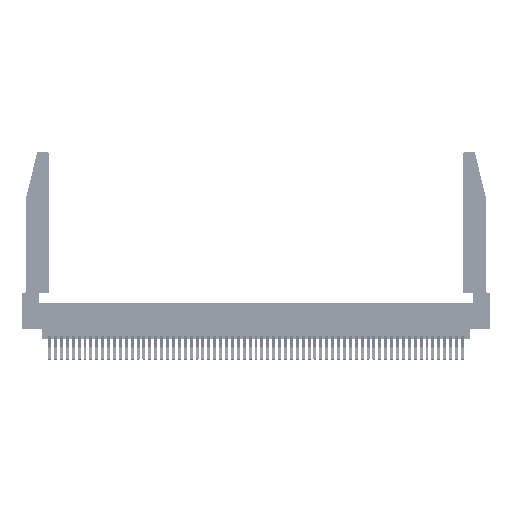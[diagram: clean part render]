
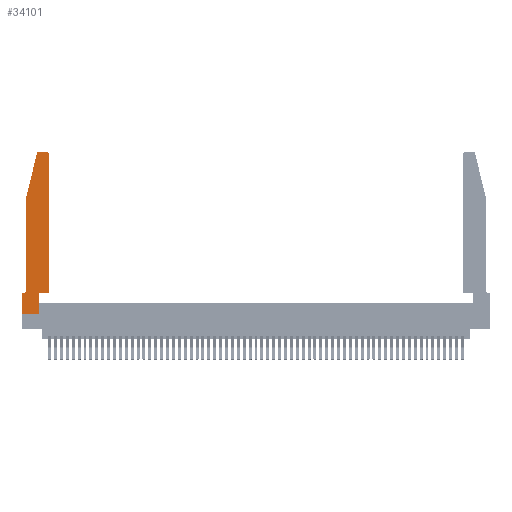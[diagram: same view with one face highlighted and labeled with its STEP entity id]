
A CAD part, top view. The second image highlights one B-rep face of the part: STEP entity #34101.
In plain terms, the highlighted planar face has unit normal (0, 0, 1).
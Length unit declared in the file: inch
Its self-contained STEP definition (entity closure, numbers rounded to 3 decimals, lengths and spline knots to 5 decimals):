
#164 = EDGE_LOOP ( 'NONE', ( #27753, #13057, #51503, #23062, #17899, #21188, #3641, #48083, #56611, #24493, #34221, #52091 ) ) ;
#1162 = LINE ( 'NONE', #53450, #11556 ) ;
#1412 = VERTEX_POINT ( 'NONE', #24696 ) ;
#2432 = CARTESIAN_POINT ( 'NONE',  ( 0.0755, 0.42, 0.37 ) ) ;
#3641 = ORIENTED_EDGE ( 'NONE', *, *, #24181, .T. ) ;
#4455 = VECTOR ( 'NONE', #11091, 39.37008 ) ;
#4553 = CARTESIAN_POINT ( 'NONE',  ( 0.4205, 2.72, 0.37 ) ) ;
#5478 = DIRECTION ( 'NONE',  ( 1., 0., 0. ) ) ;
#6006 = CARTESIAN_POINT ( 'NONE',  ( 0., 0., 0.37 ) ) ;
#6421 = EDGE_CURVE ( 'NONE', #43641, #56479, #15520, .T. ) ;
#6986 = EDGE_CURVE ( 'NONE', #33085, #43641, #43391, .T. ) ;
#7596 = DIRECTION ( 'NONE',  ( 0., 0., -1. ) ) ;
#7660 = AXIS2_PLACEMENT_3D ( 'NONE', #39767, #22393, #52934 ) ;
#7794 = VERTEX_POINT ( 'NONE', #12949 ) ;
#8035 = LINE ( 'NONE', #33126, #53197 ) ;
#8493 = VECTOR ( 'NONE', #38979, 39.37008 ) ;
#8768 = LINE ( 'NONE', #17458, #53961 ) ;
#8967 = DIRECTION ( 'NONE',  ( 1., 0., 0. ) ) ;
#10616 = LINE ( 'NONE', #17652, #33943 ) ;
#10842 = EDGE_CURVE ( 'NONE', #40890, #40761, #20466, .T. ) ;
#11091 = DIRECTION ( 'NONE',  ( 0., -1., 0. ) ) ;
#11556 = VECTOR ( 'NONE', #36266, 39.37008 ) ;
#12339 = EDGE_CURVE ( 'NONE', #35176, #49498, #49645, .T. ) ;
#12483 = EDGE_CURVE ( 'NONE', #49498, #7794, #42803, .T. ) ;
#12949 = CARTESIAN_POINT ( 'NONE',  ( 0.0055, 0.35, 0.37 ) ) ;
#13057 = ORIENTED_EDGE ( 'NONE', *, *, #10842, .T. ) ;
#15520 = CIRCLE ( 'NONE', #21879, 0.03 ) ;
#16499 = LINE ( 'NONE', #38574, #25376 ) ;
#16634 = DIRECTION ( 'NONE',  ( -1., 0., 0. ) ) ;
#16888 = DIRECTION ( 'NONE',  ( 0., 1., 0. ) ) ;
#17458 = CARTESIAN_POINT ( 'NONE',  ( 0.4505, 0.35, 0.37 ) ) ;
#17652 = CARTESIAN_POINT ( 'NONE',  ( 0., 0., 0.37 ) ) ;
#17899 = ORIENTED_EDGE ( 'NONE', *, *, #12483, .T. ) ;
#18102 = CARTESIAN_POINT ( 'NONE',  ( 0.4205, 2.75, 0.37 ) ) ;
#18366 = CARTESIAN_POINT ( 'NONE',  ( 0.284, 2.72, 0.37 ) ) ;
#18571 = CARTESIAN_POINT ( 'NONE',  ( 0., 0., 0.37 ) ) ;
#18648 = EDGE_CURVE ( 'NONE', #40761, #35176, #1162, .T. ) ;
#20393 = VECTOR ( 'NONE', #16888, 39.37008 ) ;
#20466 = CIRCLE ( 'NONE', #47632, 0.03 ) ;
#20792 = CARTESIAN_POINT ( 'NONE',  ( 0.2865, 0.35, 0.37 ) ) ;
#21188 = ORIENTED_EDGE ( 'NONE', *, *, #53151, .T. ) ;
#21415 = VERTEX_POINT ( 'NONE', #46820 ) ;
#21844 = DIRECTION ( 'NONE',  ( 1., 0., 0. ) ) ;
#21879 = AXIS2_PLACEMENT_3D ( 'NONE', #4553, #35211, #8967 ) ;
#22393 = DIRECTION ( 'NONE',  ( 0., 0., 1. ) ) ;
#22751 = DIRECTION ( 'NONE',  ( 1., 0., 0. ) ) ;
#23062 = ORIENTED_EDGE ( 'NONE', *, *, #12339, .T. ) ;
#24181 = EDGE_CURVE ( 'NONE', #21415, #53750, #10616, .T. ) ;
#24493 = ORIENTED_EDGE ( 'NONE', *, *, #51739, .T. ) ;
#24696 = CARTESIAN_POINT ( 'NONE',  ( 0.2865, 0., 0.37 ) ) ;
#25376 = VECTOR ( 'NONE', #16634, 39.37008 ) ;
#27753 = ORIENTED_EDGE ( 'NONE', *, *, #56295, .T. ) ;
#31050 = VERTEX_POINT ( 'NONE', #20792 ) ;
#32021 = LINE ( 'NONE', #42979, #20393 ) ;
#32397 = VECTOR ( 'NONE', #5478, 39.37008 ) ;
#33085 = VERTEX_POINT ( 'NONE', #36828 ) ;
#33126 = CARTESIAN_POINT ( 'NONE',  ( 0.0755, 0.35, 0.37 ) ) ;
#33766 = LINE ( 'NONE', #18571, #32397 ) ;
#33865 = CARTESIAN_POINT ( 'NONE',  ( 0.0055, 0.42, 0.37 ) ) ;
#33943 = VECTOR ( 'NONE', #48166, 39.37008 ) ;
#34101 = ADVANCED_FACE ( 'NONE', ( #39408 ), #52744, .T. ) ;
#34221 = ORIENTED_EDGE ( 'NONE', *, *, #6986, .T. ) ;
#34592 = CARTESIAN_POINT ( 'NONE',  ( 0.4505, 0.35, 0.37 ) ) ;
#35176 = VERTEX_POINT ( 'NONE', #56108 ) ;
#35211 = DIRECTION ( 'NONE',  ( 0., 0., 1. ) ) ;
#36266 = DIRECTION ( 'NONE',  ( -0.239, -0.971, 0. ) ) ;
#36828 = CARTESIAN_POINT ( 'NONE',  ( 0.4505, 0.35, 0.37 ) ) ;
#37314 = CARTESIAN_POINT ( 'NONE',  ( 0.0755, 2., 0.37 ) ) ;
#37482 = CARTESIAN_POINT ( 'NONE',  ( 0.4505, 2.72, 0.37 ) ) ;
#37518 = DIRECTION ( 'NONE',  ( -1., 0., 0. ) ) ;
#38257 = DIRECTION ( 'NONE',  ( -1., 0., 0. ) ) ;
#38574 = CARTESIAN_POINT ( 'NONE',  ( 0.2605, 2.75, 0.37 ) ) ;
#38979 = DIRECTION ( 'NONE',  ( 0., 1., 0. ) ) ;
#39335 = CARTESIAN_POINT ( 'NONE',  ( 0.25487, 2.72718, 0.37 ) ) ;
#39408 = FACE_OUTER_BOUND ( 'NONE', #164, .T. ) ;
#39767 = CARTESIAN_POINT ( 'NONE',  ( 0., 0.35, 0.37 ) ) ;
#40761 = VERTEX_POINT ( 'NONE', #39335 ) ;
#40890 = VERTEX_POINT ( 'NONE', #44437 ) ;
#42803 = CIRCLE ( 'NONE', #48042, 0.07 ) ;
#42979 = CARTESIAN_POINT ( 'NONE',  ( 0.2865, 0.35, 0.37 ) ) ;
#43391 = LINE ( 'NONE', #34592, #8493 ) ;
#43517 = EDGE_CURVE ( 'NONE', #53750, #1412, #33766, .T. ) ;
#43641 = VERTEX_POINT ( 'NONE', #37482 ) ;
#44437 = CARTESIAN_POINT ( 'NONE',  ( 0.284, 2.75, 0.37 ) ) ;
#46820 = CARTESIAN_POINT ( 'NONE',  ( 0., 0.35, 0.37 ) ) ;
#47632 = AXIS2_PLACEMENT_3D ( 'NONE', #18366, #48876, #22751 ) ;
#48042 = AXIS2_PLACEMENT_3D ( 'NONE', #33865, #7596, #38257 ) ;
#48083 = ORIENTED_EDGE ( 'NONE', *, *, #43517, .T. ) ;
#48166 = DIRECTION ( 'NONE',  ( 0., -1., 0. ) ) ;
#48876 = DIRECTION ( 'NONE',  ( 0., 0., 1. ) ) ;
#49498 = VERTEX_POINT ( 'NONE', #2432 ) ;
#49645 = LINE ( 'NONE', #37314, #4455 ) ;
#51503 = ORIENTED_EDGE ( 'NONE', *, *, #18648, .T. ) ;
#51739 = EDGE_CURVE ( 'NONE', #31050, #33085, #8768, .T. ) ;
#52091 = ORIENTED_EDGE ( 'NONE', *, *, #6421, .T. ) ;
#52744 = PLANE ( 'NONE',  #7660 ) ;
#52934 = DIRECTION ( 'NONE',  ( 1., 0., 0. ) ) ;
#53151 = EDGE_CURVE ( 'NONE', #7794, #21415, #8035, .T. ) ;
#53197 = VECTOR ( 'NONE', #37518, 39.37008 ) ;
#53351 = EDGE_CURVE ( 'NONE', #1412, #31050, #32021, .T. ) ;
#53450 = CARTESIAN_POINT ( 'NONE',  ( 0.0755, 2., 0.37 ) ) ;
#53750 = VERTEX_POINT ( 'NONE', #6006 ) ;
#53961 = VECTOR ( 'NONE', #21844, 39.37008 ) ;
#56108 = CARTESIAN_POINT ( 'NONE',  ( 0.0755, 2., 0.37 ) ) ;
#56295 = EDGE_CURVE ( 'NONE', #56479, #40890, #16499, .T. ) ;
#56479 = VERTEX_POINT ( 'NONE', #18102 ) ;
#56611 = ORIENTED_EDGE ( 'NONE', *, *, #53351, .T. ) ;
